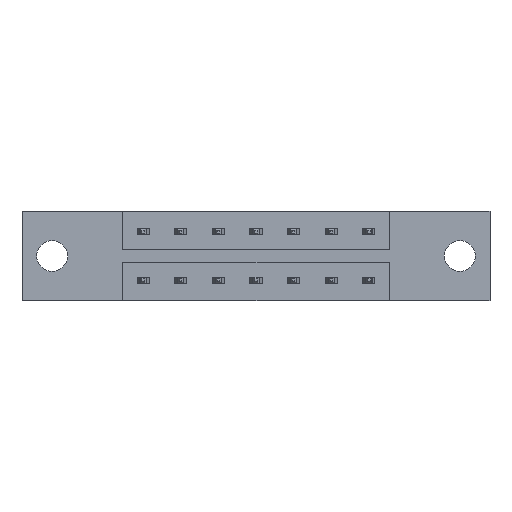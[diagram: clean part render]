
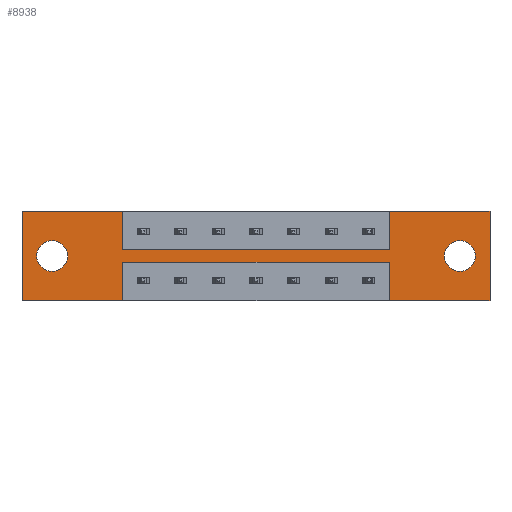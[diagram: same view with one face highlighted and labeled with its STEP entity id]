
A CAD part, front view. The second image highlights one B-rep face of the part: STEP entity #8938.
In plain terms, the highlighted planar face has unit normal (0, -1, 0).
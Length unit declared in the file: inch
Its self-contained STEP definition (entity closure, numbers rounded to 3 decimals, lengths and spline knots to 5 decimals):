
#56 = EDGE_CURVE ( 'NONE', #6536, #1837, #7971, .T. ) ;
#60 = CARTESIAN_POINT ( 'NONE',  ( 0.125, 0., -0.249 ) ) ;
#64 = DIRECTION ( 'NONE',  ( 0., 1., 0. ) ) ;
#137 = AXIS2_PLACEMENT_3D ( 'NONE', #8623, #8724, #7393 ) ;
#225 = VECTOR ( 'NONE', #6672, 39.37008 ) ;
#255 = VERTEX_POINT ( 'NONE', #5011 ) ;
#294 = ORIENTED_EDGE ( 'NONE', *, *, #7982, .T. ) ;
#302 = VECTOR ( 'NONE', #6481, 39.37008 ) ;
#325 = EDGE_CURVE ( 'NONE', #4492, #8547, #3676, .T. ) ;
#625 = VECTOR ( 'NONE', #7237, 39.37008 ) ;
#637 = CARTESIAN_POINT ( 'NONE',  ( 0.125, 0., -0.185 ) ) ;
#689 = DIRECTION ( 'NONE',  ( 0., 1., 0. ) ) ;
#704 = EDGE_CURVE ( 'NONE', #6925, #6596, #924, .T. ) ;
#728 = DIRECTION ( 'NONE',  ( 0., 0., 1. ) ) ;
#758 = DIRECTION ( 'NONE',  ( 0., 0., -1. ) ) ;
#811 = CARTESIAN_POINT ( 'NONE',  ( 0., 0., -0.37 ) ) ;
#924 = CIRCLE ( 'NONE', #2103, 0.064 ) ;
#938 = ORIENTED_EDGE ( 'NONE', *, *, #704, .T. ) ;
#1015 = VECTOR ( 'NONE', #758, 39.37008 ) ;
#1026 = CARTESIAN_POINT ( 'NONE',  ( 0., 0., -0.37 ) ) ;
#1055 = VECTOR ( 'NONE', #6519, 39.37008 ) ;
#1190 = ORIENTED_EDGE ( 'NONE', *, *, #1925, .F. ) ;
#1243 = EDGE_LOOP ( 'NONE', ( #4485, #294 ) ) ;
#1356 = CARTESIAN_POINT ( 'NONE',  ( 1.5225, 0., -0.1585 ) ) ;
#1371 = DIRECTION ( 'NONE',  ( 0., 0., 1. ) ) ;
#1378 = CARTESIAN_POINT ( 'NONE',  ( 1.5225, 0., -0.1585 ) ) ;
#1404 = ORIENTED_EDGE ( 'NONE', *, *, #2104, .T. ) ;
#1554 = ORIENTED_EDGE ( 'NONE', *, *, #3774, .F. ) ;
#1644 = PLANE ( 'NONE',  #8491 ) ;
#1705 = VECTOR ( 'NONE', #3446, 39.37008 ) ;
#1837 = VERTEX_POINT ( 'NONE', #4442 ) ;
#1925 = EDGE_CURVE ( 'NONE', #8312, #8862, #8143, .T. ) ;
#2009 = CARTESIAN_POINT ( 'NONE',  ( 0.4175, 0., 0. ) ) ;
#2103 = AXIS2_PLACEMENT_3D ( 'NONE', #637, #6239, #1371 ) ;
#2104 = EDGE_CURVE ( 'NONE', #6596, #6925, #2764, .T. ) ;
#2119 = CARTESIAN_POINT ( 'NONE',  ( 1.5225, 0., -0.2115 ) ) ;
#2228 = VECTOR ( 'NONE', #6964, 39.37008 ) ;
#2252 = VERTEX_POINT ( 'NONE', #6537 ) ;
#2268 = EDGE_CURVE ( 'NONE', #5520, #5155, #4098, .T. ) ;
#2764 = CIRCLE ( 'NONE', #7887, 0.064 ) ;
#3241 = AXIS2_PLACEMENT_3D ( 'NONE', #7047, #64, #3561 ) ;
#3446 = DIRECTION ( 'NONE',  ( 0., 0., 1. ) ) ;
#3451 = ORIENTED_EDGE ( 'NONE', *, *, #6124, .F. ) ;
#3561 = DIRECTION ( 'NONE',  ( 0., 0., -1. ) ) ;
#3676 = LINE ( 'NONE', #8958, #4603 ) ;
#3711 = LINE ( 'NONE', #8427, #1055 ) ;
#3774 = EDGE_CURVE ( 'NONE', #7504, #6536, #8097, .T. ) ;
#3793 = CARTESIAN_POINT ( 'NONE',  ( 0., 0., 0. ) ) ;
#3829 = ORIENTED_EDGE ( 'NONE', *, *, #4910, .F. ) ;
#3840 = DIRECTION ( 'NONE',  ( -1., 0., 0. ) ) ;
#3859 = FACE_BOUND ( 'NONE', #4040, .T. ) ;
#4040 = EDGE_LOOP ( 'NONE', ( #938, #1404 ) ) ;
#4098 = CIRCLE ( 'NONE', #137, 0.064 ) ;
#4335 = EDGE_CURVE ( 'NONE', #8547, #6464, #8986, .T. ) ;
#4383 = CARTESIAN_POINT ( 'NONE',  ( 0.4175, 0., -0.1585 ) ) ;
#4397 = EDGE_CURVE ( 'NONE', #8390, #2252, #3711, .T. ) ;
#4442 = CARTESIAN_POINT ( 'NONE',  ( 0.4175, 0., -0.37 ) ) ;
#4458 = LINE ( 'NONE', #3793, #625 ) ;
#4485 = ORIENTED_EDGE ( 'NONE', *, *, #2268, .T. ) ;
#4492 = VERTEX_POINT ( 'NONE', #811 ) ;
#4553 = CARTESIAN_POINT ( 'NONE',  ( 1.94, 0., 0. ) ) ;
#4562 = EDGE_CURVE ( 'NONE', #255, #5936, #4458, .T. ) ;
#4568 = CARTESIAN_POINT ( 'NONE',  ( 0., 0., 0. ) ) ;
#4603 = VECTOR ( 'NONE', #728, 39.37008 ) ;
#4631 = LINE ( 'NONE', #1026, #7873 ) ;
#4669 = CARTESIAN_POINT ( 'NONE',  ( 1.815, 0., -0.249 ) ) ;
#4686 = CARTESIAN_POINT ( 'NONE',  ( 0., 0., 0. ) ) ;
#4705 = DIRECTION ( 'NONE',  ( 1., 0., 0. ) ) ;
#4741 = VECTOR ( 'NONE', #6510, 39.37008 ) ;
#4865 = CIRCLE ( 'NONE', #3241, 0.064 ) ;
#4910 = EDGE_CURVE ( 'NONE', #2252, #7504, #4957, .T. ) ;
#4957 = LINE ( 'NONE', #2119, #1705 ) ;
#5011 = CARTESIAN_POINT ( 'NONE',  ( 1.5225, 0., 0. ) ) ;
#5080 = ORIENTED_EDGE ( 'NONE', *, *, #4397, .F. ) ;
#5082 = CARTESIAN_POINT ( 'NONE',  ( 0.4175, 0., -0.1585 ) ) ;
#5095 = FACE_BOUND ( 'NONE', #1243, .T. ) ;
#5112 = EDGE_CURVE ( 'NONE', #1837, #4492, #4631, .T. ) ;
#5155 = VERTEX_POINT ( 'NONE', #4669 ) ;
#5185 = CARTESIAN_POINT ( 'NONE',  ( 1.5225, 0., -0.2115 ) ) ;
#5195 = FACE_OUTER_BOUND ( 'NONE', #6686, .T. ) ;
#5215 = CARTESIAN_POINT ( 'NONE',  ( 0.4175, 0., -0.1585 ) ) ;
#5235 = LINE ( 'NONE', #4553, #302 ) ;
#5248 = CARTESIAN_POINT ( 'NONE',  ( 0.4175, 0., -0.2115 ) ) ;
#5320 = VECTOR ( 'NONE', #5512, 39.37008 ) ;
#5408 = ORIENTED_EDGE ( 'NONE', *, *, #4335, .F. ) ;
#5512 = DIRECTION ( 'NONE',  ( 1., 0., 0. ) ) ;
#5520 = VERTEX_POINT ( 'NONE', #8340 ) ;
#5565 = CARTESIAN_POINT ( 'NONE',  ( 0.125, 0., -0.121 ) ) ;
#5586 = CARTESIAN_POINT ( 'NONE',  ( 1.94, 0., 0. ) ) ;
#5618 = DIRECTION ( 'NONE',  ( 0., 0., 1. ) ) ;
#5798 = CARTESIAN_POINT ( 'NONE',  ( 1.94, 0., -0.37 ) ) ;
#5876 = DIRECTION ( 'NONE',  ( 0., -1., 0. ) ) ;
#5936 = VERTEX_POINT ( 'NONE', #5586 ) ;
#6124 = EDGE_CURVE ( 'NONE', #6464, #8312, #6322, .T. ) ;
#6239 = DIRECTION ( 'NONE',  ( 0., 1., 0. ) ) ;
#6322 = LINE ( 'NONE', #5082, #1015 ) ;
#6402 = ORIENTED_EDGE ( 'NONE', *, *, #7840, .F. ) ;
#6464 = VERTEX_POINT ( 'NONE', #2009 ) ;
#6481 = DIRECTION ( 'NONE',  ( 0., 0., -1. ) ) ;
#6510 = DIRECTION ( 'NONE',  ( 0., 0., -1. ) ) ;
#6519 = DIRECTION ( 'NONE',  ( -1., 0., 0. ) ) ;
#6527 = DIRECTION ( 'NONE',  ( 0., 0., -1. ) ) ;
#6536 = VERTEX_POINT ( 'NONE', #7096 ) ;
#6537 = CARTESIAN_POINT ( 'NONE',  ( 1.5225, 0., -0.37 ) ) ;
#6596 = VERTEX_POINT ( 'NONE', #60 ) ;
#6672 = DIRECTION ( 'NONE',  ( -1., 0., 0. ) ) ;
#6686 = EDGE_LOOP ( 'NONE', ( #3829, #5080, #8591, #7179, #6402, #1190, #3451, #5408, #9023, #8089, #6733, #1554 ) ) ;
#6733 = ORIENTED_EDGE ( 'NONE', *, *, #56, .F. ) ;
#6925 = VERTEX_POINT ( 'NONE', #5565 ) ;
#6964 = DIRECTION ( 'NONE',  ( 0., 0., 1. ) ) ;
#6991 = CARTESIAN_POINT ( 'NONE',  ( 0.125, 0., -0.185 ) ) ;
#7047 = CARTESIAN_POINT ( 'NONE',  ( 1.815, 0., -0.185 ) ) ;
#7096 = CARTESIAN_POINT ( 'NONE',  ( 0.4175, 0., -0.2115 ) ) ;
#7179 = ORIENTED_EDGE ( 'NONE', *, *, #4562, .F. ) ;
#7200 = CARTESIAN_POINT ( 'NONE',  ( 0., 0., -0.37 ) ) ;
#7229 = CARTESIAN_POINT ( 'NONE',  ( 0.4175, 0., -0.2115 ) ) ;
#7237 = DIRECTION ( 'NONE',  ( 1., 0., 0. ) ) ;
#7393 = DIRECTION ( 'NONE',  ( 0., 0., -1. ) ) ;
#7504 = VERTEX_POINT ( 'NONE', #5185 ) ;
#7646 = LINE ( 'NONE', #1356, #2228 ) ;
#7840 = EDGE_CURVE ( 'NONE', #8862, #255, #7646, .T. ) ;
#7873 = VECTOR ( 'NONE', #3840, 39.37008 ) ;
#7887 = AXIS2_PLACEMENT_3D ( 'NONE', #6991, #689, #5618 ) ;
#7971 = LINE ( 'NONE', #7229, #4741 ) ;
#7982 = EDGE_CURVE ( 'NONE', #5155, #5520, #4865, .T. ) ;
#8089 = ORIENTED_EDGE ( 'NONE', *, *, #5112, .F. ) ;
#8097 = LINE ( 'NONE', #5248, #225 ) ;
#8143 = LINE ( 'NONE', #5215, #8607 ) ;
#8312 = VERTEX_POINT ( 'NONE', #4383 ) ;
#8340 = CARTESIAN_POINT ( 'NONE',  ( 1.815, 0., -0.121 ) ) ;
#8390 = VERTEX_POINT ( 'NONE', #5798 ) ;
#8427 = CARTESIAN_POINT ( 'NONE',  ( 0., 0., -0.37 ) ) ;
#8491 = AXIS2_PLACEMENT_3D ( 'NONE', #7200, #5876, #6527 ) ;
#8547 = VERTEX_POINT ( 'NONE', #4568 ) ;
#8591 = ORIENTED_EDGE ( 'NONE', *, *, #8974, .F. ) ;
#8607 = VECTOR ( 'NONE', #4705, 39.37008 ) ;
#8623 = CARTESIAN_POINT ( 'NONE',  ( 1.815, 0., -0.185 ) ) ;
#8724 = DIRECTION ( 'NONE',  ( 0., 1., 0. ) ) ;
#8862 = VERTEX_POINT ( 'NONE', #1378 ) ;
#8938 = ADVANCED_FACE ( 'NONE', ( #5095, #3859, #5195 ), #1644, .T. ) ;
#8958 = CARTESIAN_POINT ( 'NONE',  ( 0., 0., 0. ) ) ;
#8974 = EDGE_CURVE ( 'NONE', #5936, #8390, #5235, .T. ) ;
#8986 = LINE ( 'NONE', #4686, #5320 ) ;
#9023 = ORIENTED_EDGE ( 'NONE', *, *, #325, .F. ) ;
